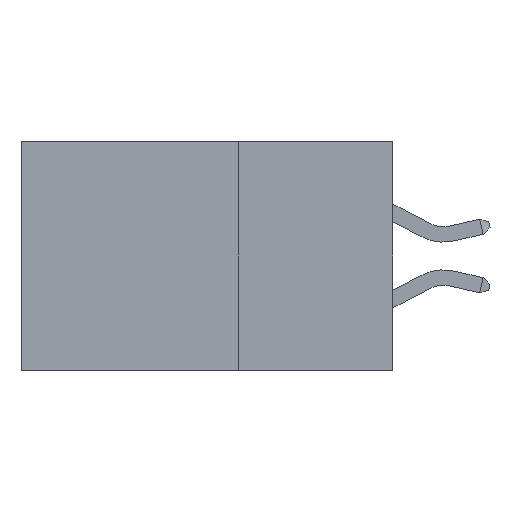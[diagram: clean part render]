
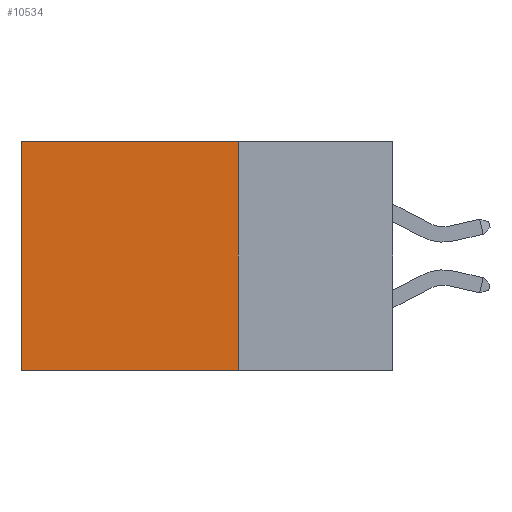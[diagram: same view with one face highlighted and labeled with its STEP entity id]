
A CAD part, left-side view. The second image highlights one B-rep face of the part: STEP entity #10534.
In plain terms, the highlighted planar face has unit normal (-1, 0, 0).
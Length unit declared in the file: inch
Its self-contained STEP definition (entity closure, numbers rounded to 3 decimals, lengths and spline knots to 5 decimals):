
#91 = VECTOR ( 'NONE', #14765, 39.37008 ) ;
#263 = CARTESIAN_POINT ( 'NONE',  ( 0.2875, 0.25, 0. ) ) ;
#602 = CARTESIAN_POINT ( 'NONE',  ( 0.2875, 0.25, 0. ) ) ;
#656 = VECTOR ( 'NONE', #1307, 39.37008 ) ;
#822 = EDGE_CURVE ( 'NONE', #9224, #10015, #1498, .T. ) ;
#1307 = DIRECTION ( 'NONE',  ( 0., 1., 0. ) ) ;
#1498 = LINE ( 'NONE', #263, #7058 ) ;
#1766 = DIRECTION ( 'NONE',  ( 1., 0., 0. ) ) ;
#2338 = CARTESIAN_POINT ( 'NONE',  ( 0.2875, 0.6, -0.37 ) ) ;
#2545 = EDGE_CURVE ( 'NONE', #8565, #3192, #4077, .T. ) ;
#2675 = DIRECTION ( 'NONE',  ( 0., 0., -1. ) ) ;
#2945 = FACE_OUTER_BOUND ( 'NONE', #13472, .T. ) ;
#2990 = EDGE_CURVE ( 'NONE', #9224, #8565, #11992, .T. ) ;
#3192 = VERTEX_POINT ( 'NONE', #2338 ) ;
#3567 = ORIENTED_EDGE ( 'NONE', *, *, #2990, .T. ) ;
#3630 = EDGE_CURVE ( 'NONE', #10015, #3192, #9659, .T. ) ;
#4077 = LINE ( 'NONE', #14678, #91 ) ;
#6280 = ORIENTED_EDGE ( 'NONE', *, *, #2545, .T. ) ;
#6954 = ORIENTED_EDGE ( 'NONE', *, *, #822, .F. ) ;
#7058 = VECTOR ( 'NONE', #2675, 39.37008 ) ;
#8043 = CARTESIAN_POINT ( 'NONE',  ( 0.2875, 0.6, 0. ) ) ;
#8211 = CARTESIAN_POINT ( 'NONE',  ( 0.2875, 0.25, -0.37 ) ) ;
#8504 = DIRECTION ( 'NONE',  ( 0., 1., 0. ) ) ;
#8565 = VERTEX_POINT ( 'NONE', #8043 ) ;
#8953 = CARTESIAN_POINT ( 'NONE',  ( 0.2875, 0.25, 0. ) ) ;
#9224 = VERTEX_POINT ( 'NONE', #602 ) ;
#9609 = VECTOR ( 'NONE', #8504, 39.37008 ) ;
#9659 = LINE ( 'NONE', #14495, #656 ) ;
#10015 = VERTEX_POINT ( 'NONE', #8211 ) ;
#10534 = ADVANCED_FACE ( 'NONE', ( #2945 ), #12459, .F. ) ;
#10901 = CARTESIAN_POINT ( 'NONE',  ( 0.2875, 0.25, 0. ) ) ;
#11992 = LINE ( 'NONE', #10901, #9609 ) ;
#12459 = PLANE ( 'NONE',  #14238 ) ;
#12538 = DIRECTION ( 'NONE',  ( 0., 0., -1. ) ) ;
#13472 = EDGE_LOOP ( 'NONE', ( #6280, #13613, #6954, #3567 ) ) ;
#13613 = ORIENTED_EDGE ( 'NONE', *, *, #3630, .F. ) ;
#14238 = AXIS2_PLACEMENT_3D ( 'NONE', #8953, #1766, #12538 ) ;
#14495 = CARTESIAN_POINT ( 'NONE',  ( 0.2875, 0.25, -0.37 ) ) ;
#14678 = CARTESIAN_POINT ( 'NONE',  ( 0.2875, 0.6, 0. ) ) ;
#14765 = DIRECTION ( 'NONE',  ( 0., 0., -1. ) ) ;
